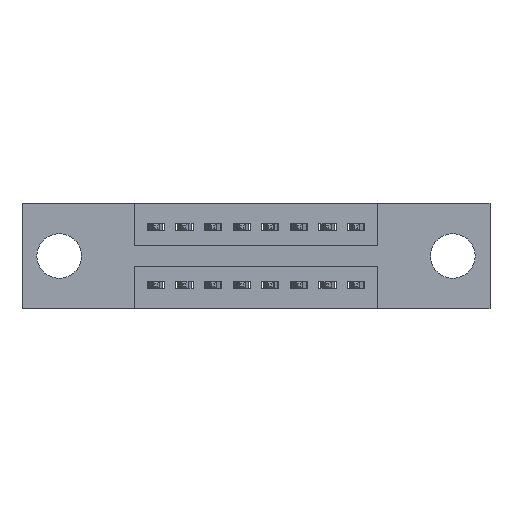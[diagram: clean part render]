
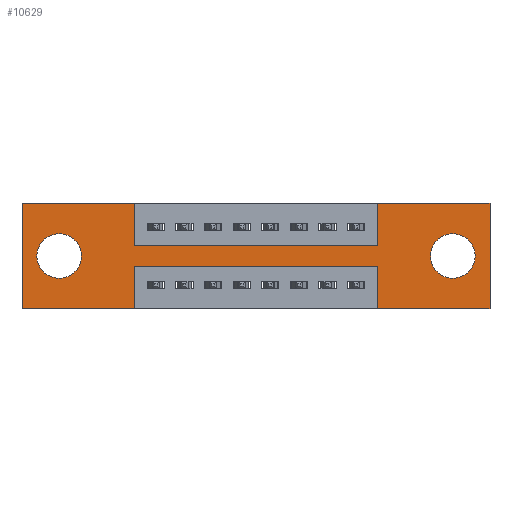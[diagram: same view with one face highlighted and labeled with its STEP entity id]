
A CAD part, front view. The second image highlights one B-rep face of the part: STEP entity #10629.
In plain terms, the highlighted planar face has unit normal (0, -1, 0).
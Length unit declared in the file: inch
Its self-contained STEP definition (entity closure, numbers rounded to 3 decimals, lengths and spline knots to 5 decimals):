
#31 = CARTESIAN_POINT ( 'NONE',  ( 0.13, 0., -0.185 ) ) ;
#60 = VECTOR ( 'NONE', #6915, 39.37008 ) ;
#76 = DIRECTION ( 'NONE',  ( 0., 1., 0. ) ) ;
#102 = CARTESIAN_POINT ( 'NONE',  ( 0.3925, 0., -0.22 ) ) ;
#281 = CARTESIAN_POINT ( 'NONE',  ( 1.2425, 0., -0.37 ) ) ;
#667 = LINE ( 'NONE', #281, #9507 ) ;
#858 = VECTOR ( 'NONE', #7808, 39.37008 ) ;
#931 = EDGE_LOOP ( 'NONE', ( #2180, #4613 ) ) ;
#932 = VERTEX_POINT ( 'NONE', #2072 ) ;
#945 = AXIS2_PLACEMENT_3D ( 'NONE', #1962, #76, #2528 ) ;
#946 = ORIENTED_EDGE ( 'NONE', *, *, #6205, .F. ) ;
#955 = ORIENTED_EDGE ( 'NONE', *, *, #9214, .F. ) ;
#958 = DIRECTION ( 'NONE',  ( 0., 0., 1. ) ) ;
#981 = ORIENTED_EDGE ( 'NONE', *, *, #6605, .F. ) ;
#991 = DIRECTION ( 'NONE',  ( -1., 0., 0. ) ) ;
#1050 = ORIENTED_EDGE ( 'NONE', *, *, #8770, .F. ) ;
#1062 = VECTOR ( 'NONE', #7922, 39.37008 ) ;
#1066 = FACE_BOUND ( 'NONE', #2677, .T. ) ;
#1216 = ORIENTED_EDGE ( 'NONE', *, *, #5341, .F. ) ;
#1224 = ORIENTED_EDGE ( 'NONE', *, *, #9338, .F. ) ;
#1286 = ORIENTED_EDGE ( 'NONE', *, *, #8584, .T. ) ;
#1330 = ORIENTED_EDGE ( 'NONE', *, *, #10302, .F. ) ;
#1421 = ORIENTED_EDGE ( 'NONE', *, *, #3596, .F. ) ;
#1426 = ORIENTED_EDGE ( 'NONE', *, *, #4989, .F. ) ;
#1560 = CARTESIAN_POINT ( 'NONE',  ( 0.3925, 0., -0.15 ) ) ;
#1651 = CARTESIAN_POINT ( 'NONE',  ( 0., 0., 0. ) ) ;
#1660 = EDGE_CURVE ( 'NONE', #9025, #932, #10529, .T. ) ;
#1778 = VERTEX_POINT ( 'NONE', #5753 ) ;
#1821 = VERTEX_POINT ( 'NONE', #5269 ) ;
#1856 = CARTESIAN_POINT ( 'NONE',  ( 0., 0., -0.37 ) ) ;
#1951 = VERTEX_POINT ( 'NONE', #9303 ) ;
#1959 = LINE ( 'NONE', #5250, #8521 ) ;
#1962 = CARTESIAN_POINT ( 'NONE',  ( 0.13, 0., -0.185 ) ) ;
#1997 = DIRECTION ( 'NONE',  ( 0., 0., 1. ) ) ;
#2024 = LINE ( 'NONE', #8162, #10626 ) ;
#2051 = ORIENTED_EDGE ( 'NONE', *, *, #10545, .F. ) ;
#2072 = CARTESIAN_POINT ( 'NONE',  ( 0.13, 0., -0.263 ) ) ;
#2142 = LINE ( 'NONE', #1651, #4177 ) ;
#2180 = ORIENTED_EDGE ( 'NONE', *, *, #5730, .T. ) ;
#2223 = DIRECTION ( 'NONE',  ( 0., 1., 0. ) ) ;
#2425 = LINE ( 'NONE', #10149, #60 ) ;
#2528 = DIRECTION ( 'NONE',  ( 0., 0., 1. ) ) ;
#2657 = VERTEX_POINT ( 'NONE', #8942 ) ;
#2677 = EDGE_LOOP ( 'NONE', ( #2744, #1286 ) ) ;
#2678 = EDGE_CURVE ( 'NONE', #7040, #1778, #8604, .T. ) ;
#2744 = ORIENTED_EDGE ( 'NONE', *, *, #1660, .T. ) ;
#2834 = CARTESIAN_POINT ( 'NONE',  ( 0.3925, 0., -0.22 ) ) ;
#2835 = DIRECTION ( 'NONE',  ( 0., 0., -1. ) ) ;
#2842 = DIRECTION ( 'NONE',  ( 0., 1., 0. ) ) ;
#2844 = CARTESIAN_POINT ( 'NONE',  ( 1.505, 0., -0.185 ) ) ;
#2912 = ORIENTED_EDGE ( 'NONE', *, *, #2678, .F. ) ;
#2982 = VERTEX_POINT ( 'NONE', #5640 ) ;
#3334 = CARTESIAN_POINT ( 'NONE',  ( 0., 0., -0.37 ) ) ;
#3357 = LINE ( 'NONE', #102, #1062 ) ;
#3497 = ORIENTED_EDGE ( 'NONE', *, *, #7252, .F. ) ;
#3519 = DIRECTION ( 'NONE',  ( 0., 0., -1. ) ) ;
#3596 = EDGE_CURVE ( 'NONE', #4022, #2657, #2024, .T. ) ;
#3793 = AXIS2_PLACEMENT_3D ( 'NONE', #2844, #2842, #2835 ) ;
#4022 = VERTEX_POINT ( 'NONE', #1560 ) ;
#4075 = VECTOR ( 'NONE', #1997, 39.37008 ) ;
#4177 = VECTOR ( 'NONE', #9358, 39.37008 ) ;
#4316 = VERTEX_POINT ( 'NONE', #8306 ) ;
#4401 = DIRECTION ( 'NONE',  ( -1., 0., 0. ) ) ;
#4613 = ORIENTED_EDGE ( 'NONE', *, *, #9838, .T. ) ;
#4886 = CIRCLE ( 'NONE', #8601, 0.078 ) ;
#4918 = LINE ( 'NONE', #1856, #9175 ) ;
#4989 = EDGE_CURVE ( 'NONE', #8064, #4022, #7771, .T. ) ;
#5112 = CIRCLE ( 'NONE', #7799, 0.078 ) ;
#5136 = DIRECTION ( 'NONE',  ( 0., 0., 1. ) ) ;
#5137 = VERTEX_POINT ( 'NONE', #6904 ) ;
#5224 = PLANE ( 'NONE',  #7737 ) ;
#5250 = CARTESIAN_POINT ( 'NONE',  ( 1.2425, 0., 0. ) ) ;
#5269 = CARTESIAN_POINT ( 'NONE',  ( 1.635, 0., -0.37 ) ) ;
#5302 = VERTEX_POINT ( 'NONE', #5683 ) ;
#5341 = EDGE_CURVE ( 'NONE', #2657, #5137, #1959, .T. ) ;
#5501 = DIRECTION ( 'NONE',  ( 0., 0., 1. ) ) ;
#5640 = CARTESIAN_POINT ( 'NONE',  ( 1.505, 0., -0.263 ) ) ;
#5683 = CARTESIAN_POINT ( 'NONE',  ( 1.635, 0., 0. ) ) ;
#5730 = EDGE_CURVE ( 'NONE', #4316, #2982, #9788, .T. ) ;
#5753 = CARTESIAN_POINT ( 'NONE',  ( 0., 0., 0. ) ) ;
#5951 = FACE_BOUND ( 'NONE', #931, .T. ) ;
#6104 = CARTESIAN_POINT ( 'NONE',  ( 0., 0., -0.37 ) ) ;
#6147 = DIRECTION ( 'NONE',  ( 0., 1., 0. ) ) ;
#6205 = EDGE_CURVE ( 'NONE', #5137, #5302, #10009, .T. ) ;
#6259 = CARTESIAN_POINT ( 'NONE',  ( 1.2425, 0., -0.22 ) ) ;
#6404 = VECTOR ( 'NONE', #4401, 39.37008 ) ;
#6605 = EDGE_CURVE ( 'NONE', #1821, #1951, #8118, .T. ) ;
#6612 = CARTESIAN_POINT ( 'NONE',  ( 0., 0., 0. ) ) ;
#6904 = CARTESIAN_POINT ( 'NONE',  ( 1.2425, 0., 0. ) ) ;
#6915 = DIRECTION ( 'NONE',  ( 0., 0., -1. ) ) ;
#6960 = CARTESIAN_POINT ( 'NONE',  ( 0.3925, 0., -0.37 ) ) ;
#7040 = VERTEX_POINT ( 'NONE', #3334 ) ;
#7252 = EDGE_CURVE ( 'NONE', #10630, #7040, #4918, .T. ) ;
#7320 = VERTEX_POINT ( 'NONE', #6259 ) ;
#7402 = CARTESIAN_POINT ( 'NONE',  ( 1.505, 0., -0.185 ) ) ;
#7691 = FACE_OUTER_BOUND ( 'NONE', #9971, .T. ) ;
#7737 = AXIS2_PLACEMENT_3D ( 'NONE', #6104, #8644, #3519 ) ;
#7771 = LINE ( 'NONE', #7833, #858 ) ;
#7799 = AXIS2_PLACEMENT_3D ( 'NONE', #7402, #2223, #8233 ) ;
#7808 = DIRECTION ( 'NONE',  ( 0., 0., -1. ) ) ;
#7833 = CARTESIAN_POINT ( 'NONE',  ( 0.3925, 0., 0. ) ) ;
#7922 = DIRECTION ( 'NONE',  ( -1., 0., 0. ) ) ;
#8032 = VERTEX_POINT ( 'NONE', #2834 ) ;
#8050 = CARTESIAN_POINT ( 'NONE',  ( 0., 0., 0. ) ) ;
#8064 = VERTEX_POINT ( 'NONE', #10376 ) ;
#8118 = LINE ( 'NONE', #9491, #6404 ) ;
#8136 = DIRECTION ( 'NONE',  ( 1., 0., 0. ) ) ;
#8162 = CARTESIAN_POINT ( 'NONE',  ( 0.3925, 0., -0.15 ) ) ;
#8206 = DIRECTION ( 'NONE',  ( 1., 0., 0. ) ) ;
#8233 = DIRECTION ( 'NONE',  ( 0., 0., -1. ) ) ;
#8306 = CARTESIAN_POINT ( 'NONE',  ( 1.505, 0., -0.107 ) ) ;
#8307 = VECTOR ( 'NONE', #9692, 39.37008 ) ;
#8521 = VECTOR ( 'NONE', #5136, 39.37008 ) ;
#8556 = LINE ( 'NONE', #8892, #8307 ) ;
#8584 = EDGE_CURVE ( 'NONE', #932, #9025, #4886, .T. ) ;
#8601 = AXIS2_PLACEMENT_3D ( 'NONE', #31, #6147, #958 ) ;
#8604 = LINE ( 'NONE', #6612, #4075 ) ;
#8644 = DIRECTION ( 'NONE',  ( 0., -1., 0. ) ) ;
#8770 = EDGE_CURVE ( 'NONE', #1951, #7320, #667, .T. ) ;
#8892 = CARTESIAN_POINT ( 'NONE',  ( 0.3925, 0., -0.37 ) ) ;
#8942 = CARTESIAN_POINT ( 'NONE',  ( 1.2425, 0., -0.15 ) ) ;
#9025 = VERTEX_POINT ( 'NONE', #9942 ) ;
#9175 = VECTOR ( 'NONE', #991, 39.37008 ) ;
#9214 = EDGE_CURVE ( 'NONE', #5302, #1821, #2425, .T. ) ;
#9303 = CARTESIAN_POINT ( 'NONE',  ( 1.2425, 0., -0.37 ) ) ;
#9338 = EDGE_CURVE ( 'NONE', #7320, #8032, #3357, .T. ) ;
#9358 = DIRECTION ( 'NONE',  ( 1., 0., 0. ) ) ;
#9491 = CARTESIAN_POINT ( 'NONE',  ( 0., 0., -0.37 ) ) ;
#9507 = VECTOR ( 'NONE', #5501, 39.37008 ) ;
#9692 = DIRECTION ( 'NONE',  ( 0., 0., -1. ) ) ;
#9788 = CIRCLE ( 'NONE', #3793, 0.078 ) ;
#9838 = EDGE_CURVE ( 'NONE', #2982, #4316, #5112, .T. ) ;
#9942 = CARTESIAN_POINT ( 'NONE',  ( 0.13, 0., -0.107 ) ) ;
#9971 = EDGE_LOOP ( 'NONE', ( #1330, #1224, #1050, #981, #955, #946, #1216, #1421, #1426, #2051, #2912, #3497 ) ) ;
#10009 = LINE ( 'NONE', #8050, #10219 ) ;
#10149 = CARTESIAN_POINT ( 'NONE',  ( 1.635, 0., 0. ) ) ;
#10219 = VECTOR ( 'NONE', #8136, 39.37008 ) ;
#10302 = EDGE_CURVE ( 'NONE', #8032, #10630, #8556, .T. ) ;
#10376 = CARTESIAN_POINT ( 'NONE',  ( 0.3925, 0., 0. ) ) ;
#10529 = CIRCLE ( 'NONE', #945, 0.078 ) ;
#10545 = EDGE_CURVE ( 'NONE', #1778, #8064, #2142, .T. ) ;
#10626 = VECTOR ( 'NONE', #8206, 39.37008 ) ;
#10629 = ADVANCED_FACE ( 'NONE', ( #5951, #1066, #7691 ), #5224, .T. ) ;
#10630 = VERTEX_POINT ( 'NONE', #6960 ) ;
